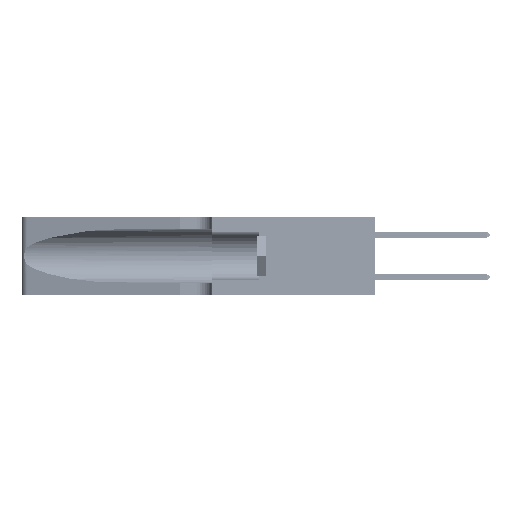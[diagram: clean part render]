
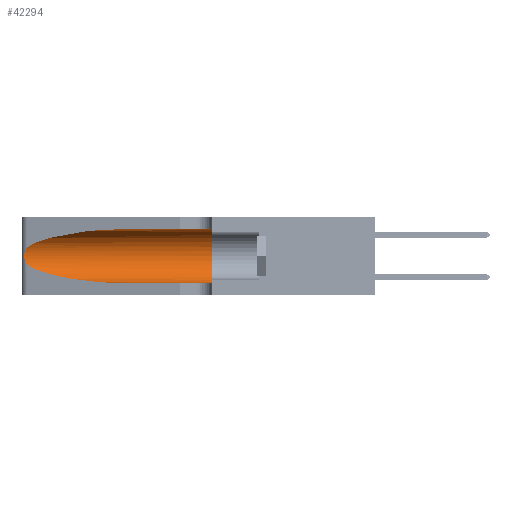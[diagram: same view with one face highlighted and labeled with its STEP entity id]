
A CAD part, left-side view. The second image highlights one B-rep face of the part: STEP entity #42294.
In plain terms, the highlighted cylindrical face has radius 3.308 mm (diameter 6.617 mm), a partial arc.
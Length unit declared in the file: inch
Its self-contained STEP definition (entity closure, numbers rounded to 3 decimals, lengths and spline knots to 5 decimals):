
#182 = CARTESIAN_POINT ( 'NONE',  ( 0.1305, 0.72297, 0.05475 ) ) ;
#1079 = VERTEX_POINT ( 'NONE', #42153 ) ;
#3120 = CYLINDRICAL_SURFACE ( 'NONE', #18005, 0.13025 ) ;
#3480 = EDGE_LOOP ( 'NONE', ( #42938, #41946, #41052, #30121, #53589, #47430 ) ) ;
#4224 = CARTESIAN_POINT ( 'NONE',  ( 0.26075, 1.23896, 0.19203 ) ) ;
#5616 = CIRCLE ( 'NONE', #46747, 0.13025 ) ;
#6709 = VECTOR ( 'NONE', #12818, 39.37008 ) ;
#7196 = DIRECTION ( 'NONE',  ( 0., 1., 0. ) ) ;
#7293 = DIRECTION ( 'NONE',  ( 0., 0., -1. ) ) ;
#8542 = CARTESIAN_POINT ( 'NONE',  ( 0.26017, 1.23833, 0.17102 ) ) ;
#8572 = CARTESIAN_POINT ( 'NONE',  ( 0.1305, 1.61858, 0.05475 ) ) ;
#9604 = CARTESIAN_POINT ( 'NONE',  ( 0.1305, 0.72297, 0.31525 ) ) ;
#11525 = DIRECTION ( 'NONE',  ( 0., -1., 0. ) ) ;
#12698 = CARTESIAN_POINT ( 'NONE',  ( 0.25487, 1.22718, 0.22369 ) ) ;
#12792 = CARTESIAN_POINT ( 'NONE',  ( 0.25789, 1.23486, 0.15765 ) ) ;
#12818 = DIRECTION ( 'NONE',  ( 0., -1., 0. ) ) ;
#13824 = CARTESIAN_POINT ( 'NONE',  ( 0.1305, 0.72297, 0.31525 ) ) ;
#14160 =( BOUNDED_CURVE ( )  B_SPLINE_CURVE ( 3, ( #13824, #26598, #43494, #18257 ),
 .UNSPECIFIED., .F., .F. ) 
 B_SPLINE_CURVE_WITH_KNOTS ( ( 4, 4 ),
 ( 1.5708, 2.84003 ),
 .UNSPECIFIED. ) 
 CURVE ( )  GEOMETRIC_REPRESENTATION_ITEM ( )  RATIONAL_B_SPLINE_CURVE ( ( 1., 0.87, 0.87, 1. ) ) 
 REPRESENTATION_ITEM ( '' )  );
#16535 = LINE ( 'NONE', #53409, #26441 ) ;
#16871 = CARTESIAN_POINT ( 'NONE',  ( 0.25487, 1.22718, 0.22369 ) ) ;
#17046 = CARTESIAN_POINT ( 'NONE',  ( 0.25555, 1.22993, 0.14849 ) ) ;
#18005 = AXIS2_PLACEMENT_3D ( 'NONE', #36808, #11525, #7293 ) ;
#18233 =( BOUNDED_CURVE ( )  B_SPLINE_CURVE ( 3, ( #49551, #24325, #53776, #28608 ),
 .UNSPECIFIED., .F., .F. ) 
 B_SPLINE_CURVE_WITH_KNOTS ( ( 4, 4 ),
 ( 3.44316, 4.71239 ),
 .UNSPECIFIED. ) 
 CURVE ( )  GEOMETRIC_REPRESENTATION_ITEM ( )  RATIONAL_B_SPLINE_CURVE ( ( 1., 0.87, 0.87, 1. ) ) 
 REPRESENTATION_ITEM ( '' )  );
#18257 = CARTESIAN_POINT ( 'NONE',  ( 0.25487, 1.22718, 0.22369 ) ) ;
#21001 = EDGE_CURVE ( 'NONE', #26621, #46730, #16535, .T. ) ;
#21788 = VERTEX_POINT ( 'NONE', #12698 ) ;
#24325 = CARTESIAN_POINT ( 'NONE',  ( 0.2373, 1.15595, 0.08982 ) ) ;
#25373 = CARTESIAN_POINT ( 'NONE',  ( 0.1305, 0.35, 0.31525 ) ) ;
#25376 = CARTESIAN_POINT ( 'NONE',  ( 0.25787, 1.23484, 0.2124 ) ) ;
#26441 = VECTOR ( 'NONE', #40702, 39.37008 ) ;
#26598 = CARTESIAN_POINT ( 'NONE',  ( 0.18966, 0.96281, 0.31525 ) ) ;
#26621 = VERTEX_POINT ( 'NONE', #9604 ) ;
#28608 = CARTESIAN_POINT ( 'NONE',  ( 0.1305, 0.72297, 0.05475 ) ) ;
#29623 = CARTESIAN_POINT ( 'NONE',  ( 0.26018, 1.23835, 0.19895 ) ) ;
#30121 = ORIENTED_EDGE ( 'NONE', *, *, #50547, .T. ) ;
#30523 = LINE ( 'NONE', #8572, #6709 ) ;
#31035 = EDGE_CURVE ( 'NONE', #21788, #1079, #37842, .T. ) ;
#32514 = CARTESIAN_POINT ( 'NONE',  ( 0.1305, 0.35, 0.185 ) ) ;
#33831 = CARTESIAN_POINT ( 'NONE',  ( 0.26075, 1.23896, 0.178 ) ) ;
#34992 = EDGE_CURVE ( 'NONE', #1079, #49352, #18233, .T. ) ;
#36720 = DIRECTION ( 'NONE',  ( 0., 0., 1. ) ) ;
#36808 = CARTESIAN_POINT ( 'NONE',  ( 0.1305, 1.61858, 0.185 ) ) ;
#37842 = B_SPLINE_CURVE_WITH_KNOTS ( 'NONE', 3,
 ( #16871, #42098, #50575, #25376, #46810, #29623, #4224, #33831, #8542, #38043, #12792, #42279, #17046, #46527 ),
 .UNSPECIFIED., .F., .F.,
 ( 4, 2, 2, 2, 2, 2, 4 ),
 ( 0., 0.00027, 0.00053, 0.00107, 0.0016, 0.00187, 0.00214 ),
 .UNSPECIFIED. ) ;
#38043 = CARTESIAN_POINT ( 'NONE',  ( 0.25856, 1.23593, 0.16098 ) ) ;
#40702 = DIRECTION ( 'NONE',  ( 0., -1., 0. ) ) ;
#41052 = ORIENTED_EDGE ( 'NONE', *, *, #34992, .T. ) ;
#41946 = ORIENTED_EDGE ( 'NONE', *, *, #31035, .T. ) ;
#42098 = CARTESIAN_POINT ( 'NONE',  ( 0.25555, 1.22994, 0.2215 ) ) ;
#42153 = CARTESIAN_POINT ( 'NONE',  ( 0.25487, 1.22718, 0.14631 ) ) ;
#42279 = CARTESIAN_POINT ( 'NONE',  ( 0.25639, 1.23186, 0.15144 ) ) ;
#42294 = ADVANCED_FACE ( 'NONE', ( #48063 ), #3120, .F. ) ;
#42938 = ORIENTED_EDGE ( 'NONE', *, *, #51408, .T. ) ;
#43494 = CARTESIAN_POINT ( 'NONE',  ( 0.2373, 1.15595, 0.28018 ) ) ;
#46527 = CARTESIAN_POINT ( 'NONE',  ( 0.25487, 1.22718, 0.14631 ) ) ;
#46730 = VERTEX_POINT ( 'NONE', #25373 ) ;
#46747 = AXIS2_PLACEMENT_3D ( 'NONE', #32514, #7196, #36720 ) ;
#46810 = CARTESIAN_POINT ( 'NONE',  ( 0.25854, 1.2359, 0.20912 ) ) ;
#47430 = ORIENTED_EDGE ( 'NONE', *, *, #21001, .F. ) ;
#48063 = FACE_OUTER_BOUND ( 'NONE', #3480, .T. ) ;
#49352 = VERTEX_POINT ( 'NONE', #182 ) ;
#49551 = CARTESIAN_POINT ( 'NONE',  ( 0.25487, 1.22718, 0.14631 ) ) ;
#50547 = EDGE_CURVE ( 'NONE', #49352, #50687, #30523, .T. ) ;
#50575 = CARTESIAN_POINT ( 'NONE',  ( 0.25639, 1.23184, 0.21858 ) ) ;
#50687 = VERTEX_POINT ( 'NONE', #51481 ) ;
#51408 = EDGE_CURVE ( 'NONE', #26621, #21788, #14160, .T. ) ;
#51481 = CARTESIAN_POINT ( 'NONE',  ( 0.1305, 0.35, 0.05475 ) ) ;
#53409 = CARTESIAN_POINT ( 'NONE',  ( 0.1305, 1.61858, 0.31525 ) ) ;
#53589 = ORIENTED_EDGE ( 'NONE', *, *, #53931, .F. ) ;
#53776 = CARTESIAN_POINT ( 'NONE',  ( 0.18966, 0.96281, 0.05475 ) ) ;
#53931 = EDGE_CURVE ( 'NONE', #46730, #50687, #5616, .T. ) ;
